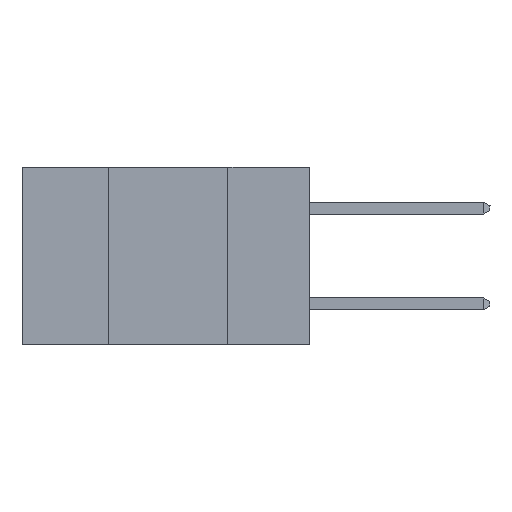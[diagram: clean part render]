
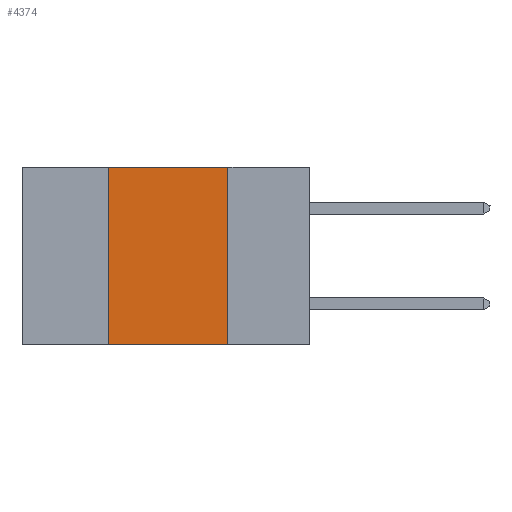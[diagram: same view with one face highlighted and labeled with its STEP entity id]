
A CAD part, left-side view. The second image highlights one B-rep face of the part: STEP entity #4374.
In plain terms, the highlighted planar face has unit normal (-1, 0, 0).
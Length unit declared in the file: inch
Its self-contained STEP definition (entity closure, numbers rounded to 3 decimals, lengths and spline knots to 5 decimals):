
#938 = EDGE_LOOP ( 'NONE', ( #20068, #5983, #19090, #21440 ) ) ;
#1495 = VERTEX_POINT ( 'NONE', #15506 ) ;
#2359 = PLANE ( 'NONE',  #15726 ) ;
#3571 = CARTESIAN_POINT ( 'NONE',  ( 0., 0.17, 0. ) ) ;
#4271 = DIRECTION ( 'NONE',  ( 0., 0., -1. ) ) ;
#4374 = ADVANCED_FACE ( 'NONE', ( #19508 ), #2359, .F. ) ;
#4809 = CARTESIAN_POINT ( 'NONE',  ( 0., 0.6, -0.37 ) ) ;
#5983 = ORIENTED_EDGE ( 'NONE', *, *, #23555, .F. ) ;
#6273 = LINE ( 'NONE', #12149, #8418 ) ;
#6359 = DIRECTION ( 'NONE',  ( 0., 0., 1. ) ) ;
#6746 = CARTESIAN_POINT ( 'NONE',  ( 0., 0.42, 0. ) ) ;
#6984 = DIRECTION ( 'NONE',  ( 0., -1., 0. ) ) ;
#7123 = DIRECTION ( 'NONE',  ( 0., 0., -1. ) ) ;
#7954 = LINE ( 'NONE', #4809, #18612 ) ;
#8418 = VECTOR ( 'NONE', #6359, 39.37008 ) ;
#9231 = EDGE_CURVE ( 'NONE', #1495, #11210, #7954, .T. ) ;
#9619 = VERTEX_POINT ( 'NONE', #3571 ) ;
#9850 = EDGE_CURVE ( 'NONE', #9619, #11210, #10308, .T. ) ;
#10308 = LINE ( 'NONE', #13999, #16137 ) ;
#11149 = CARTESIAN_POINT ( 'NONE',  ( 0., 0.6, 0. ) ) ;
#11210 = VERTEX_POINT ( 'NONE', #16971 ) ;
#12149 = CARTESIAN_POINT ( 'NONE',  ( 0., 0.42, 0. ) ) ;
#12768 = EDGE_CURVE ( 'NONE', #1495, #23409, #6273, .T. ) ;
#13999 = CARTESIAN_POINT ( 'NONE',  ( 0., 0.17, 0. ) ) ;
#15506 = CARTESIAN_POINT ( 'NONE',  ( 0., 0.42, -0.37 ) ) ;
#15726 = AXIS2_PLACEMENT_3D ( 'NONE', #24084, #16019, #4271 ) ;
#15814 = VECTOR ( 'NONE', #18943, 39.37008 ) ;
#16019 = DIRECTION ( 'NONE',  ( 1., 0., 0. ) ) ;
#16137 = VECTOR ( 'NONE', #7123, 39.37008 ) ;
#16971 = CARTESIAN_POINT ( 'NONE',  ( 0., 0.17, -0.37 ) ) ;
#18612 = VECTOR ( 'NONE', #6984, 39.37008 ) ;
#18943 = DIRECTION ( 'NONE',  ( 0., -1., 0. ) ) ;
#19090 = ORIENTED_EDGE ( 'NONE', *, *, #12768, .F. ) ;
#19508 = FACE_OUTER_BOUND ( 'NONE', #938, .T. ) ;
#19785 = LINE ( 'NONE', #11149, #15814 ) ;
#20068 = ORIENTED_EDGE ( 'NONE', *, *, #9850, .F. ) ;
#21440 = ORIENTED_EDGE ( 'NONE', *, *, #9231, .T. ) ;
#23409 = VERTEX_POINT ( 'NONE', #6746 ) ;
#23555 = EDGE_CURVE ( 'NONE', #23409, #9619, #19785, .T. ) ;
#24084 = CARTESIAN_POINT ( 'NONE',  ( 0., 0.6, 0. ) ) ;
